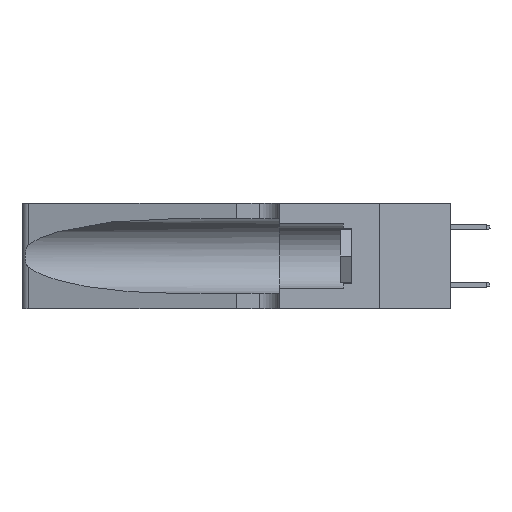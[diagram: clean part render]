
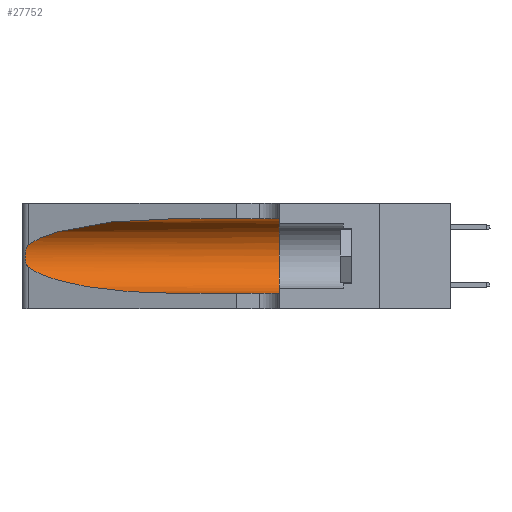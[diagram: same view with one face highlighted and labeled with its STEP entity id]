
A CAD part, left-side view. The second image highlights one B-rep face of the part: STEP entity #27752.
In plain terms, the highlighted cylindrical face has radius 3.308 mm (diameter 6.617 mm), a partial arc.
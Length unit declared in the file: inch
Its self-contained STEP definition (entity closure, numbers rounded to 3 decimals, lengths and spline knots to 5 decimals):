
#52 = VERTEX_POINT ( 'NONE', #13047 ) ;
#415 = CARTESIAN_POINT ( 'NONE',  ( 0.25789, 1.23486, 0.15765 ) ) ;
#1421 = ORIENTED_EDGE ( 'NONE', *, *, #10264, .T. ) ;
#1491 = ORIENTED_EDGE ( 'NONE', *, *, #11636, .T. ) ;
#2909 = CARTESIAN_POINT ( 'NONE',  ( 0.1305, 0.72297, 0.05475 ) ) ;
#3362 = EDGE_CURVE ( 'NONE', #4827, #28374, #30117, .T. ) ;
#3410 = CARTESIAN_POINT ( 'NONE',  ( 0.18966, 0.96281, 0.05475 ) ) ;
#3444 = VERTEX_POINT ( 'NONE', #9021 ) ;
#4375 = LINE ( 'NONE', #32967, #17477 ) ;
#4827 = VERTEX_POINT ( 'NONE', #24963 ) ;
#5477 = CARTESIAN_POINT ( 'NONE',  ( 0.25555, 1.22993, 0.14849 ) ) ;
#5695 = CARTESIAN_POINT ( 'NONE',  ( 0.25487, 1.22718, 0.14631 ) ) ;
#5828 = CARTESIAN_POINT ( 'NONE',  ( 0.25555, 1.22994, 0.2215 ) ) ;
#5983 = CARTESIAN_POINT ( 'NONE',  ( 0.26017, 1.23833, 0.17102 ) ) ;
#7121 = VECTOR ( 'NONE', #20570, 39.37008 ) ;
#7571 = DIRECTION ( 'NONE',  ( 0., -1., 0. ) ) ;
#8014 = CARTESIAN_POINT ( 'NONE',  ( 0.26075, 1.23896, 0.19203 ) ) ;
#8397 = ORIENTED_EDGE ( 'NONE', *, *, #15522, .F. ) ;
#8745 = ORIENTED_EDGE ( 'NONE', *, *, #3362, .T. ) ;
#9021 = CARTESIAN_POINT ( 'NONE',  ( 0.1305, 0.35, 0.05475 ) ) ;
#10099 = AXIS2_PLACEMENT_3D ( 'NONE', #28606, #7571, #10461 ) ;
#10125 = LINE ( 'NONE', #13180, #7121 ) ;
#10264 = EDGE_CURVE ( 'NONE', #23531, #4827, #16884, .T. ) ;
#10461 = DIRECTION ( 'NONE',  ( 0., 0., -1. ) ) ;
#10559 = AXIS2_PLACEMENT_3D ( 'NONE', #13270, #23971, #18769 ) ;
#11636 = EDGE_CURVE ( 'NONE', #52, #3444, #10125, .T. ) ;
#12190 =( BOUNDED_CURVE ( )  B_SPLINE_CURVE ( 3, ( #18732, #28988, #3410, #2909 ),
 .UNSPECIFIED., .F., .F. ) 
 B_SPLINE_CURVE_WITH_KNOTS ( ( 4, 4 ),
 ( 3.44316, 4.71239 ),
 .UNSPECIFIED. ) 
 CURVE ( )  GEOMETRIC_REPRESENTATION_ITEM ( )  RATIONAL_B_SPLINE_CURVE ( ( 1., 0.87, 0.87, 1. ) ) 
 REPRESENTATION_ITEM ( '' )  );
#12652 = CARTESIAN_POINT ( 'NONE',  ( 0.1305, 0.72297, 0.31525 ) ) ;
#13041 = VERTEX_POINT ( 'NONE', #21187 ) ;
#13047 = CARTESIAN_POINT ( 'NONE',  ( 0.1305, 0.72297, 0.05475 ) ) ;
#13127 = CARTESIAN_POINT ( 'NONE',  ( 0.25487, 1.22718, 0.22369 ) ) ;
#13180 = CARTESIAN_POINT ( 'NONE',  ( 0.1305, 1.61858, 0.05475 ) ) ;
#13270 = CARTESIAN_POINT ( 'NONE',  ( 0.1305, 0.35, 0.185 ) ) ;
#13899 = EDGE_CURVE ( 'NONE', #23531, #13041, #4375, .T. ) ;
#15204 = FACE_OUTER_BOUND ( 'NONE', #17478, .T. ) ;
#15522 = EDGE_CURVE ( 'NONE', #13041, #3444, #27205, .T. ) ;
#15792 = CARTESIAN_POINT ( 'NONE',  ( 0.25487, 1.22718, 0.14631 ) ) ;
#16884 =( BOUNDED_CURVE ( )  B_SPLINE_CURVE ( 3, ( #12652, #28080, #30957, #28246 ),
 .UNSPECIFIED., .F., .T. ) 
 B_SPLINE_CURVE_WITH_KNOTS ( ( 4, 4 ),
 ( 1.5708, 2.84003 ),
 .UNSPECIFIED. ) 
 CURVE ( )  GEOMETRIC_REPRESENTATION_ITEM ( )  RATIONAL_B_SPLINE_CURVE ( ( 1., 0.87, 0.87, 1. ) ) 
 REPRESENTATION_ITEM ( '' )  );
#17016 = DIRECTION ( 'NONE',  ( 0., -1., 0. ) ) ;
#17477 = VECTOR ( 'NONE', #17016, 39.37008 ) ;
#17478 = EDGE_LOOP ( 'NONE', ( #1421, #8745, #24281, #1491, #8397, #25408 ) ) ;
#18284 = CARTESIAN_POINT ( 'NONE',  ( 0.25856, 1.23593, 0.16098 ) ) ;
#18732 = CARTESIAN_POINT ( 'NONE',  ( 0.25487, 1.22718, 0.14631 ) ) ;
#18769 = DIRECTION ( 'NONE',  ( 0., 0., 1. ) ) ;
#19233 = EDGE_CURVE ( 'NONE', #28374, #52, #12190, .T. ) ;
#20570 = DIRECTION ( 'NONE',  ( 0., -1., 0. ) ) ;
#20666 = CARTESIAN_POINT ( 'NONE',  ( 0.25787, 1.23484, 0.2124 ) ) ;
#21187 = CARTESIAN_POINT ( 'NONE',  ( 0.1305, 0.35, 0.31525 ) ) ;
#23308 = CARTESIAN_POINT ( 'NONE',  ( 0.25854, 1.2359, 0.20912 ) ) ;
#23531 = VERTEX_POINT ( 'NONE', #28587 ) ;
#23971 = DIRECTION ( 'NONE',  ( 0., 1., 0. ) ) ;
#24281 = ORIENTED_EDGE ( 'NONE', *, *, #19233, .T. ) ;
#24963 = CARTESIAN_POINT ( 'NONE',  ( 0.25487, 1.22718, 0.22369 ) ) ;
#25408 = ORIENTED_EDGE ( 'NONE', *, *, #13899, .F. ) ;
#27205 = CIRCLE ( 'NONE', #10559, 0.13025 ) ;
#27752 = ADVANCED_FACE ( 'NONE', ( #15204 ), #28452, .F. ) ;
#28080 = CARTESIAN_POINT ( 'NONE',  ( 0.18966, 0.96281, 0.31525 ) ) ;
#28246 = CARTESIAN_POINT ( 'NONE',  ( 0.25487, 1.22718, 0.22369 ) ) ;
#28374 = VERTEX_POINT ( 'NONE', #5695 ) ;
#28452 = CYLINDRICAL_SURFACE ( 'NONE', #10099, 0.13025 ) ;
#28535 = CARTESIAN_POINT ( 'NONE',  ( 0.25639, 1.23186, 0.15144 ) ) ;
#28587 = CARTESIAN_POINT ( 'NONE',  ( 0.1305, 0.72297, 0.31525 ) ) ;
#28606 = CARTESIAN_POINT ( 'NONE',  ( 0.1305, 1.61858, 0.185 ) ) ;
#28703 = CARTESIAN_POINT ( 'NONE',  ( 0.25639, 1.23184, 0.21858 ) ) ;
#28988 = CARTESIAN_POINT ( 'NONE',  ( 0.2373, 1.15595, 0.08982 ) ) ;
#29034 = CARTESIAN_POINT ( 'NONE',  ( 0.26075, 1.23896, 0.178 ) ) ;
#30117 = B_SPLINE_CURVE_WITH_KNOTS ( 'NONE', 3,
 ( #13127, #5828, #28703, #20666, #23308, #31096, #8014, #29034, #5983, #18284, #415, #28535, #5477, #15792 ),
 .UNSPECIFIED., .F., .F.,
 ( 4, 2, 2, 2, 2, 2, 4 ),
 ( 0., 0.00027, 0.00053, 0.00107, 0.0016, 0.00187, 0.00214 ),
 .UNSPECIFIED. ) ;
#30957 = CARTESIAN_POINT ( 'NONE',  ( 0.2373, 1.15595, 0.28018 ) ) ;
#31096 = CARTESIAN_POINT ( 'NONE',  ( 0.26018, 1.23835, 0.19895 ) ) ;
#32967 = CARTESIAN_POINT ( 'NONE',  ( 0.1305, 1.61858, 0.31525 ) ) ;
